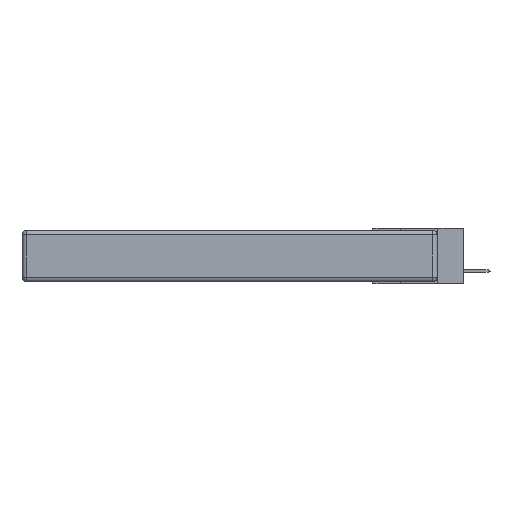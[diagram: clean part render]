
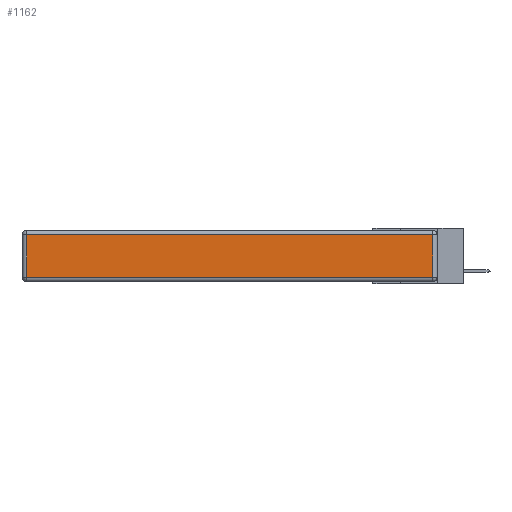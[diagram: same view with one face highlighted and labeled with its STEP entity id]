
A CAD part, left-side view. The second image highlights one B-rep face of the part: STEP entity #1162.
In plain terms, the highlighted planar face has unit normal (-1, 0, 0).
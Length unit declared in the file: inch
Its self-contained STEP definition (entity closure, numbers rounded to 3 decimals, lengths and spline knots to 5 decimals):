
#524 = AXIS2_PLACEMENT_3D ( 'NONE', #12454, #956, #4757 ) ;
#580 = EDGE_LOOP ( 'NONE', ( #18598, #20640, #23681, #10236 ) ) ;
#956 = DIRECTION ( 'NONE',  ( -1., 0., 0. ) ) ;
#1162 = ADVANCED_FACE ( 'NONE', ( #9324 ), #12381, .T. ) ;
#1796 = VECTOR ( 'NONE', #18405, 39.37008 ) ;
#2262 = VERTEX_POINT ( 'NONE', #10452 ) ;
#2750 = EDGE_CURVE ( 'NONE', #10136, #15304, #21941, .T. ) ;
#3979 = CARTESIAN_POINT ( 'NONE',  ( 0., 2.72, -0.03 ) ) ;
#4757 = DIRECTION ( 'NONE',  ( 0., 0., 1. ) ) ;
#5303 = CARTESIAN_POINT ( 'NONE',  ( 0., 0., -0.313 ) ) ;
#7571 = CARTESIAN_POINT ( 'NONE',  ( 0., 0.03, -0.03 ) ) ;
#8006 = VERTEX_POINT ( 'NONE', #12424 ) ;
#8113 = EDGE_CURVE ( 'NONE', #8006, #2262, #23707, .T. ) ;
#8967 = CARTESIAN_POINT ( 'NONE',  ( 0., 0.03, -0.343 ) ) ;
#9324 = FACE_OUTER_BOUND ( 'NONE', #580, .T. ) ;
#10136 = VERTEX_POINT ( 'NONE', #7571 ) ;
#10236 = ORIENTED_EDGE ( 'NONE', *, *, #22629, .T. ) ;
#10452 = CARTESIAN_POINT ( 'NONE',  ( 0., 0.03, -0.313 ) ) ;
#12381 = PLANE ( 'NONE',  #524 ) ;
#12424 = CARTESIAN_POINT ( 'NONE',  ( 0., 2.72, -0.313 ) ) ;
#12454 = CARTESIAN_POINT ( 'NONE',  ( 0., 0., -0.343 ) ) ;
#14776 = CARTESIAN_POINT ( 'NONE',  ( 0., 2.72, -0.343 ) ) ;
#15207 = VECTOR ( 'NONE', #21784, 39.37008 ) ;
#15304 = VERTEX_POINT ( 'NONE', #3979 ) ;
#15826 = LINE ( 'NONE', #8967, #16436 ) ;
#16436 = VECTOR ( 'NONE', #18254, 39.37008 ) ;
#16510 = EDGE_CURVE ( 'NONE', #2262, #10136, #15826, .T. ) ;
#18058 = LINE ( 'NONE', #14776, #1796 ) ;
#18254 = DIRECTION ( 'NONE',  ( 0., 0., 1. ) ) ;
#18405 = DIRECTION ( 'NONE',  ( 0., 0., -1. ) ) ;
#18598 = ORIENTED_EDGE ( 'NONE', *, *, #8113, .T. ) ;
#20640 = ORIENTED_EDGE ( 'NONE', *, *, #16510, .T. ) ;
#21784 = DIRECTION ( 'NONE',  ( 0., 1., 0. ) ) ;
#21941 = LINE ( 'NONE', #23177, #15207 ) ;
#22629 = EDGE_CURVE ( 'NONE', #15304, #8006, #18058, .T. ) ;
#23177 = CARTESIAN_POINT ( 'NONE',  ( 0., 2.75, -0.03 ) ) ;
#23681 = ORIENTED_EDGE ( 'NONE', *, *, #2750, .T. ) ;
#23707 = LINE ( 'NONE', #5303, #24012 ) ;
#23962 = DIRECTION ( 'NONE',  ( 0., -1., 0. ) ) ;
#24012 = VECTOR ( 'NONE', #23962, 39.37008 ) ;
